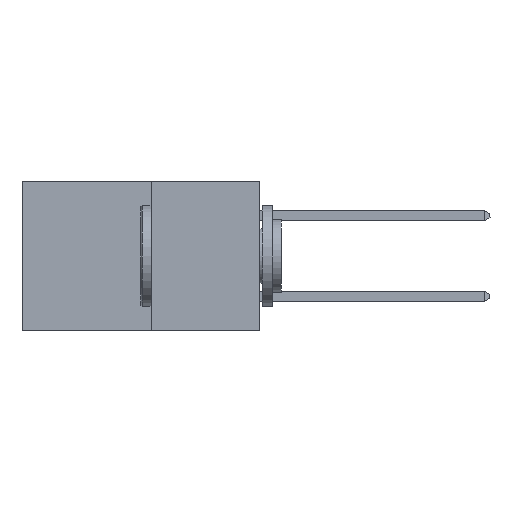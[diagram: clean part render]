
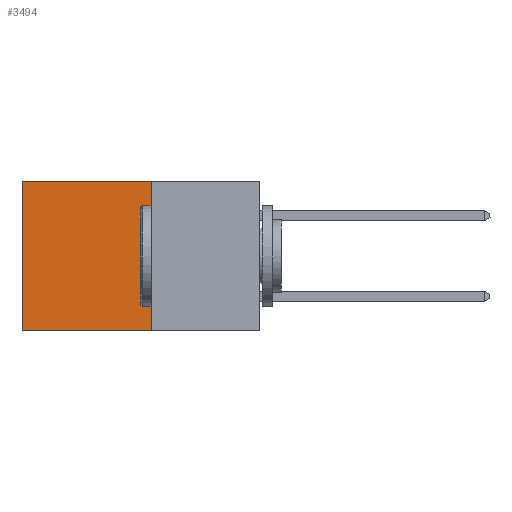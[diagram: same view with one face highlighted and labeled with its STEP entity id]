
A CAD part, left-side view. The second image highlights one B-rep face of the part: STEP entity #3494.
In plain terms, the highlighted planar face has unit normal (-1, 0, 0).
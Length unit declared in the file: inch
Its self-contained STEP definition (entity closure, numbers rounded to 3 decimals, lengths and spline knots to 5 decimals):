
#14 = CARTESIAN_POINT ( 'NONE',  ( 0.277, 0.27, -0.37 ) ) ;
#169 = CARTESIAN_POINT ( 'NONE',  ( 0.277, 0.59, -0.37 ) ) ;
#832 = CARTESIAN_POINT ( 'NONE',  ( 0.277, 0.59, 0. ) ) ;
#1372 = VECTOR ( 'NONE', #6624, 39.37008 ) ;
#1668 = LINE ( 'NONE', #5610, #6907 ) ;
#2110 = FACE_OUTER_BOUND ( 'NONE', #2614, .T. ) ;
#2282 = ORIENTED_EDGE ( 'NONE', *, *, #6082, .T. ) ;
#2614 = EDGE_LOOP ( 'NONE', ( #4990, #7113, #5595, #2282 ) ) ;
#2669 = VERTEX_POINT ( 'NONE', #832 ) ;
#3233 = DIRECTION ( 'NONE',  ( 1., 0., 0. ) ) ;
#3283 = VERTEX_POINT ( 'NONE', #4085 ) ;
#3442 = DIRECTION ( 'NONE',  ( 0., 0., -1. ) ) ;
#3494 = ADVANCED_FACE ( 'NONE', ( #2110 ), #4521, .F. ) ;
#3596 = CARTESIAN_POINT ( 'NONE',  ( 0.277, 0.27, -0.37 ) ) ;
#4085 = CARTESIAN_POINT ( 'NONE',  ( 0.277, 0.27, 0. ) ) ;
#4521 = PLANE ( 'NONE',  #8021 ) ;
#4674 = VECTOR ( 'NONE', #5508, 39.37008 ) ;
#4874 = LINE ( 'NONE', #169, #4674 ) ;
#4990 = ORIENTED_EDGE ( 'NONE', *, *, #7949, .T. ) ;
#5195 = CARTESIAN_POINT ( 'NONE',  ( 0.277, 0.27, -0.37 ) ) ;
#5508 = DIRECTION ( 'NONE',  ( 0., 0., -1. ) ) ;
#5595 = ORIENTED_EDGE ( 'NONE', *, *, #6552, .F. ) ;
#5610 = CARTESIAN_POINT ( 'NONE',  ( 0.277, 0.27, 0. ) ) ;
#5621 = VERTEX_POINT ( 'NONE', #3596 ) ;
#6082 = EDGE_CURVE ( 'NONE', #3283, #2669, #1668, .T. ) ;
#6221 = DIRECTION ( 'NONE',  ( 0., 1., 0. ) ) ;
#6336 = LINE ( 'NONE', #14, #7964 ) ;
#6409 = CARTESIAN_POINT ( 'NONE',  ( 0.277, 0.59, -0.37 ) ) ;
#6552 = EDGE_CURVE ( 'NONE', #3283, #5621, #6336, .T. ) ;
#6624 = DIRECTION ( 'NONE',  ( 0., 1., 0. ) ) ;
#6627 = LINE ( 'NONE', #6746, #1372 ) ;
#6700 = EDGE_CURVE ( 'NONE', #5621, #8269, #6627, .T. ) ;
#6746 = CARTESIAN_POINT ( 'NONE',  ( 0.277, 0.27, -0.37 ) ) ;
#6907 = VECTOR ( 'NONE', #6221, 39.37008 ) ;
#7113 = ORIENTED_EDGE ( 'NONE', *, *, #6700, .F. ) ;
#7949 = EDGE_CURVE ( 'NONE', #2669, #8269, #4874, .T. ) ;
#7964 = VECTOR ( 'NONE', #8389, 39.37008 ) ;
#8021 = AXIS2_PLACEMENT_3D ( 'NONE', #5195, #3233, #3442 ) ;
#8269 = VERTEX_POINT ( 'NONE', #6409 ) ;
#8389 = DIRECTION ( 'NONE',  ( 0., 0., -1. ) ) ;
